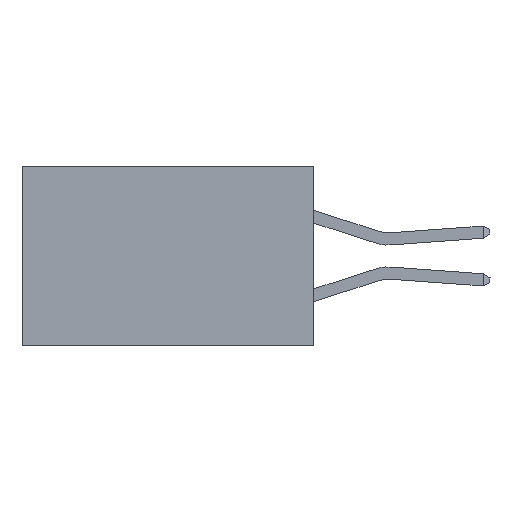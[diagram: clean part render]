
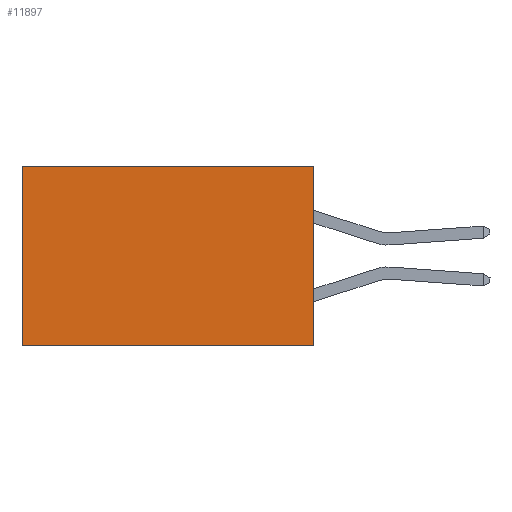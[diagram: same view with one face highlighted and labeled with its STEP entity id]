
A CAD part, left-side view. The second image highlights one B-rep face of the part: STEP entity #11897.
In plain terms, the highlighted planar face has unit normal (-1, 0, 0).
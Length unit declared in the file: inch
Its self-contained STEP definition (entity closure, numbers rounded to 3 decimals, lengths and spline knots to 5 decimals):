
#1383 = CARTESIAN_POINT ( 'NONE',  ( 0.2875, 0.6, -0.37 ) ) ;
#1596 = VECTOR ( 'NONE', #5859, 39.37008 ) ;
#2633 = LINE ( 'NONE', #21935, #1596 ) ;
#2960 = AXIS2_PLACEMENT_3D ( 'NONE', #35872, #6429, #26076 ) ;
#3964 = CARTESIAN_POINT ( 'NONE',  ( 0.2875, 0., 0. ) ) ;
#5859 = DIRECTION ( 'NONE',  ( 0., 0., -1. ) ) ;
#6045 = VECTOR ( 'NONE', #17758, 39.37008 ) ;
#6088 = VECTOR ( 'NONE', #36751, 39.37008 ) ;
#6429 = DIRECTION ( 'NONE',  ( 1., 0., 0. ) ) ;
#6539 = EDGE_LOOP ( 'NONE', ( #20002, #28013, #30015, #34998 ) ) ;
#6727 = CARTESIAN_POINT ( 'NONE',  ( 0.2875, 0.6, 0. ) ) ;
#9500 = EDGE_CURVE ( 'NONE', #28001, #30163, #14275, .T. ) ;
#9661 = EDGE_CURVE ( 'NONE', #11976, #31966, #14777, .T. ) ;
#11897 = ADVANCED_FACE ( 'NONE', ( #14977 ), #32412, .F. ) ;
#11976 = VERTEX_POINT ( 'NONE', #3964 ) ;
#14165 = CARTESIAN_POINT ( 'NONE',  ( 0.2875, 0., 0. ) ) ;
#14275 = LINE ( 'NONE', #39748, #6088 ) ;
#14777 = LINE ( 'NONE', #14165, #6045 ) ;
#14977 = FACE_OUTER_BOUND ( 'NONE', #6539, .T. ) ;
#17758 = DIRECTION ( 'NONE',  ( 0., 1., 0. ) ) ;
#18742 = VECTOR ( 'NONE', #26793, 39.37008 ) ;
#18949 = EDGE_CURVE ( 'NONE', #11976, #28001, #2633, .T. ) ;
#20002 = ORIENTED_EDGE ( 'NONE', *, *, #42514, .T. ) ;
#20035 = CARTESIAN_POINT ( 'NONE',  ( 0.2875, 0.6, 0. ) ) ;
#21935 = CARTESIAN_POINT ( 'NONE',  ( 0.2875, 0., 0. ) ) ;
#22335 = LINE ( 'NONE', #6727, #18742 ) ;
#22839 = CARTESIAN_POINT ( 'NONE',  ( 0.2875, 0., -0.37 ) ) ;
#26076 = DIRECTION ( 'NONE',  ( 0., 0., -1. ) ) ;
#26793 = DIRECTION ( 'NONE',  ( 0., 0., -1. ) ) ;
#28001 = VERTEX_POINT ( 'NONE', #22839 ) ;
#28013 = ORIENTED_EDGE ( 'NONE', *, *, #9500, .F. ) ;
#30015 = ORIENTED_EDGE ( 'NONE', *, *, #18949, .F. ) ;
#30163 = VERTEX_POINT ( 'NONE', #1383 ) ;
#31966 = VERTEX_POINT ( 'NONE', #20035 ) ;
#32412 = PLANE ( 'NONE',  #2960 ) ;
#34998 = ORIENTED_EDGE ( 'NONE', *, *, #9661, .T. ) ;
#35872 = CARTESIAN_POINT ( 'NONE',  ( 0.2875, 0., 0. ) ) ;
#36751 = DIRECTION ( 'NONE',  ( 0., 1., 0. ) ) ;
#39748 = CARTESIAN_POINT ( 'NONE',  ( 0.2875, 0., -0.37 ) ) ;
#42514 = EDGE_CURVE ( 'NONE', #31966, #30163, #22335, .T. ) ;
